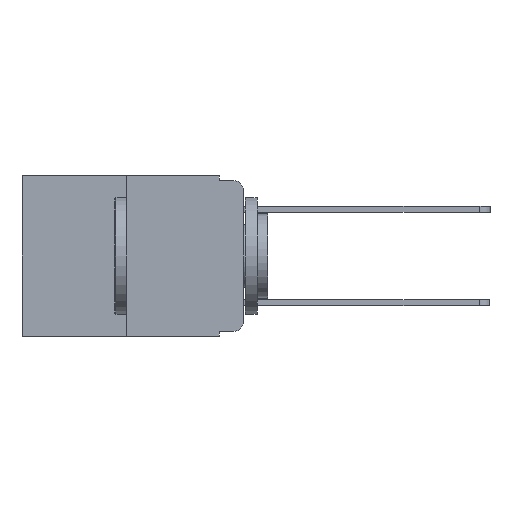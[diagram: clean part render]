
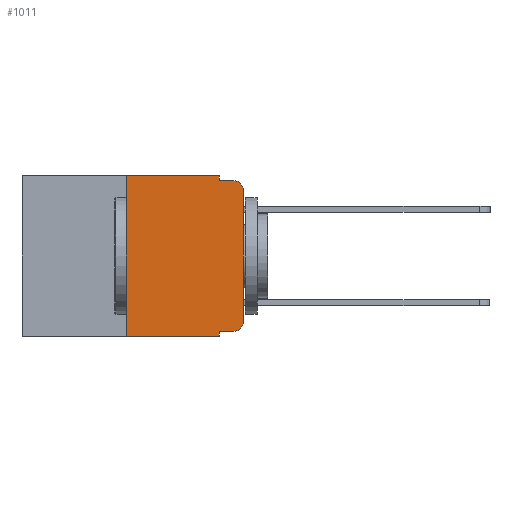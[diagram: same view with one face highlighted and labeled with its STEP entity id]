
A CAD part, left-side view. The second image highlights one B-rep face of the part: STEP entity #1011.
In plain terms, the highlighted planar face has unit normal (-1, 0, 0).
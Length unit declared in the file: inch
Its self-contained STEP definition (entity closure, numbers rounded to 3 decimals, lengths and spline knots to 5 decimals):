
#107 = DIRECTION ( 'NONE',  ( 0., -1., 0. ) ) ;
#184 = EDGE_CURVE ( 'NONE', #5621, #10835, #252, .T. ) ;
#252 = LINE ( 'NONE', #13415, #10670 ) ;
#308 = CIRCLE ( 'NONE', #8951, 0.02 ) ;
#472 = CARTESIAN_POINT ( 'NONE',  ( 0., 0.051, -0.01 ) ) ;
#1011 = ADVANCED_FACE ( 'NONE', ( #5460 ), #14692, .F. ) ;
#1568 = DIRECTION ( 'NONE',  ( -1., 0., 0. ) ) ;
#2011 = CARTESIAN_POINT ( 'NONE',  ( 0., 0., -0.03 ) ) ;
#2106 = CARTESIAN_POINT ( 'NONE',  ( 0., 0.02, -0.01 ) ) ;
#2413 = CARTESIAN_POINT ( 'NONE',  ( 0., 0.051, -0.01 ) ) ;
#2574 = EDGE_CURVE ( 'NONE', #12680, #8345, #3537, .T. ) ;
#3441 = EDGE_CURVE ( 'NONE', #8345, #7791, #13935, .T. ) ;
#3537 = LINE ( 'NONE', #9134, #16105 ) ;
#3593 = LINE ( 'NONE', #2413, #12868 ) ;
#3865 = CARTESIAN_POINT ( 'NONE',  ( 0., 0.473, -0.343 ) ) ;
#4315 = VECTOR ( 'NONE', #14527, 39.37008 ) ;
#5069 = DIRECTION ( 'NONE',  ( 0., -1., 0. ) ) ;
#5405 = CARTESIAN_POINT ( 'NONE',  ( 0., 0.02, -0.313 ) ) ;
#5460 = FACE_OUTER_BOUND ( 'NONE', #6969, .T. ) ;
#5558 = CARTESIAN_POINT ( 'NONE',  ( 0., 0.051, -0.333 ) ) ;
#5621 = VERTEX_POINT ( 'NONE', #13669 ) ;
#5714 = DIRECTION ( 'NONE',  ( 0., 0., -1. ) ) ;
#6694 = DIRECTION ( 'NONE',  ( 0., 0., -1. ) ) ;
#6932 = LINE ( 'NONE', #3865, #10313 ) ;
#6949 = EDGE_CURVE ( 'NONE', #14017, #5621, #16068, .T. ) ;
#6969 = EDGE_LOOP ( 'NONE', ( #11765, #11900, #12015, #12192, #12269, #12420, #12432, #12436, #12815, #12830 ) ) ;
#7171 = CARTESIAN_POINT ( 'NONE',  ( 0., 0., 0. ) ) ;
#7445 = CARTESIAN_POINT ( 'NONE',  ( 0., 0.25, 0. ) ) ;
#7715 = EDGE_CURVE ( 'NONE', #14017, #9720, #6932, .T. ) ;
#7791 = VERTEX_POINT ( 'NONE', #11599 ) ;
#8230 = DIRECTION ( 'NONE',  ( 0., 0., -1. ) ) ;
#8267 = CARTESIAN_POINT ( 'NONE',  ( 0., 0.051, 0. ) ) ;
#8345 = VERTEX_POINT ( 'NONE', #8941 ) ;
#8681 = EDGE_CURVE ( 'NONE', #12680, #9720, #14799, .T. ) ;
#8735 = DIRECTION ( 'NONE',  ( 0., 0., 1. ) ) ;
#8941 = CARTESIAN_POINT ( 'NONE',  ( 0., 0.02, -0.333 ) ) ;
#8951 = AXIS2_PLACEMENT_3D ( 'NONE', #9399, #1568, #10643 ) ;
#9134 = CARTESIAN_POINT ( 'NONE',  ( 0., 0.051, -0.333 ) ) ;
#9399 = CARTESIAN_POINT ( 'NONE',  ( 0., 0.02, -0.03 ) ) ;
#9502 = CARTESIAN_POINT ( 'NONE',  ( 0., 0.051, 0. ) ) ;
#9720 = VERTEX_POINT ( 'NONE', #11072 ) ;
#9781 = CARTESIAN_POINT ( 'NONE',  ( 0., 0.25, -0.343 ) ) ;
#10313 = VECTOR ( 'NONE', #12697, 39.37008 ) ;
#10429 = VECTOR ( 'NONE', #5714, 39.37008 ) ;
#10643 = DIRECTION ( 'NONE',  ( 0., 0., -1. ) ) ;
#10670 = VECTOR ( 'NONE', #13251, 39.37008 ) ;
#10835 = VERTEX_POINT ( 'NONE', #13116 ) ;
#11025 = VERTEX_POINT ( 'NONE', #2011 ) ;
#11072 = CARTESIAN_POINT ( 'NONE',  ( 0., 0.051, -0.343 ) ) ;
#11102 = LINE ( 'NONE', #7171, #4315 ) ;
#11173 = EDGE_CURVE ( 'NONE', #14632, #11709, #3593, .T. ) ;
#11599 = CARTESIAN_POINT ( 'NONE',  ( 0., 0., -0.313 ) ) ;
#11609 = VECTOR ( 'NONE', #8230, 39.37008 ) ;
#11709 = VERTEX_POINT ( 'NONE', #2106 ) ;
#11765 = ORIENTED_EDGE ( 'NONE', *, *, #15215, .T. ) ;
#11900 = ORIENTED_EDGE ( 'NONE', *, *, #16080, .T. ) ;
#12015 = ORIENTED_EDGE ( 'NONE', *, *, #11173, .F. ) ;
#12192 = ORIENTED_EDGE ( 'NONE', *, *, #12765, .F. ) ;
#12269 = ORIENTED_EDGE ( 'NONE', *, *, #184, .F. ) ;
#12420 = ORIENTED_EDGE ( 'NONE', *, *, #6949, .F. ) ;
#12432 = ORIENTED_EDGE ( 'NONE', *, *, #7715, .T. ) ;
#12436 = ORIENTED_EDGE ( 'NONE', *, *, #8681, .F. ) ;
#12680 = VERTEX_POINT ( 'NONE', #5558 ) ;
#12697 = DIRECTION ( 'NONE',  ( 0., -1., 0. ) ) ;
#12765 = EDGE_CURVE ( 'NONE', #10835, #14632, #13626, .T. ) ;
#12770 = AXIS2_PLACEMENT_3D ( 'NONE', #14823, #14672, #14649 ) ;
#12781 = VECTOR ( 'NONE', #8735, 39.37008 ) ;
#12815 = ORIENTED_EDGE ( 'NONE', *, *, #2574, .T. ) ;
#12830 = ORIENTED_EDGE ( 'NONE', *, *, #3441, .T. ) ;
#12868 = VECTOR ( 'NONE', #5069, 39.37008 ) ;
#13116 = CARTESIAN_POINT ( 'NONE',  ( 0., 0.051, 0. ) ) ;
#13251 = DIRECTION ( 'NONE',  ( 0., -1., 0. ) ) ;
#13415 = CARTESIAN_POINT ( 'NONE',  ( 0., 0.473, 0. ) ) ;
#13626 = LINE ( 'NONE', #8267, #10429 ) ;
#13669 = CARTESIAN_POINT ( 'NONE',  ( 0., 0.25, 0. ) ) ;
#13935 = CIRCLE ( 'NONE', #15689, 0.02 ) ;
#14017 = VERTEX_POINT ( 'NONE', #9781 ) ;
#14092 = DIRECTION ( 'NONE',  ( -1., 0., 0. ) ) ;
#14527 = DIRECTION ( 'NONE',  ( 0., 0., 1. ) ) ;
#14632 = VERTEX_POINT ( 'NONE', #472 ) ;
#14649 = DIRECTION ( 'NONE',  ( 0., 0., -1. ) ) ;
#14672 = DIRECTION ( 'NONE',  ( 1., 0., 0. ) ) ;
#14692 = PLANE ( 'NONE',  #12770 ) ;
#14799 = LINE ( 'NONE', #9502, #11609 ) ;
#14823 = CARTESIAN_POINT ( 'NONE',  ( 0., 0.473, 0. ) ) ;
#15215 = EDGE_CURVE ( 'NONE', #7791, #11025, #11102, .T. ) ;
#15689 = AXIS2_PLACEMENT_3D ( 'NONE', #5405, #14092, #6694 ) ;
#16068 = LINE ( 'NONE', #7445, #12781 ) ;
#16080 = EDGE_CURVE ( 'NONE', #11025, #11709, #308, .T. ) ;
#16105 = VECTOR ( 'NONE', #107, 39.37008 ) ;
